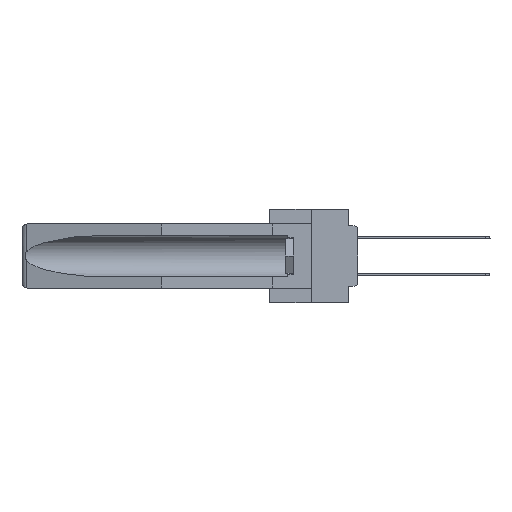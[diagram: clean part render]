
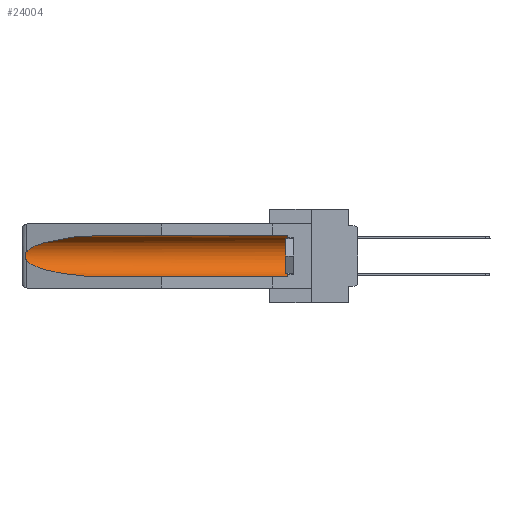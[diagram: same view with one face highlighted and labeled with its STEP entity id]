
A CAD part, left-side view. The second image highlights one B-rep face of the part: STEP entity #24004.
In plain terms, the highlighted cylindrical face has radius 2.857 mm (diameter 5.715 mm), a partial arc.
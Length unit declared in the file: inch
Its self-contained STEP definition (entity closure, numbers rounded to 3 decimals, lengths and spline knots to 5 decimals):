
#847 = CARTESIAN_POINT ( 'NONE',  ( 0.26537, 1.52718, -0.14972 ) ) ;
#1030 = CARTESIAN_POINT ( 'NONE',  ( 0.26654, 1.53092, -0.15636 ) ) ;
#1283 = CARTESIAN_POINT ( 'NONE',  ( 0.21114, 1.30732, -0.059 ) ) ;
#1475 = CARTESIAN_POINT ( 'NONE',  ( 0.2675, 1.53308, -0.16763 ) ) ;
#3165 = VERTEX_POINT ( 'NONE', #23333 ) ;
#3193 = DIRECTION ( 'NONE',  ( 0., 1., 0. ) ) ;
#3310 = B_SPLINE_CURVE_WITH_KNOTS ( 'NONE', 3,
 ( #15070, #26556, #1030, #21716, #1475, #8117, #28674, #17335, #8264, #5844 ),
 .UNSPECIFIED., .F., .F.,
 ( 4, 2, 2, 2, 4 ),
 ( 0., 0.00029, 0.00058, 0.00087, 0.00117 ),
 .UNSPECIFIED. ) ;
#3900 = CARTESIAN_POINT ( 'NONE',  ( 0.155, 0.126, -0.1715 ) ) ;
#3917 = CARTESIAN_POINT ( 'NONE',  ( 0.26537, 1.52718, -0.19328 ) ) ;
#4339 = VERTEX_POINT ( 'NONE', #29647 ) ;
#4673 = EDGE_CURVE ( 'NONE', #3165, #19928, #6039, .T. ) ;
#5576 = VECTOR ( 'NONE', #3193, 39.37008 ) ;
#5599 = VERTEX_POINT ( 'NONE', #15603 ) ;
#5844 = CARTESIAN_POINT ( 'NONE',  ( 0.26537, 1.52718, -0.19328 ) ) ;
#5873 = CARTESIAN_POINT ( 'NONE',  ( 0.25451, 1.48313, -0.24835 ) ) ;
#6039 = LINE ( 'NONE', #24465, #5576 ) ;
#6092 = FACE_OUTER_BOUND ( 'NONE', #16623, .T. ) ;
#7738 = ORIENTED_EDGE ( 'NONE', *, *, #23647, .T. ) ;
#7782 = CARTESIAN_POINT ( 'NONE',  ( 0.25451, 1.48313, -0.09465 ) ) ;
#7866 = VERTEX_POINT ( 'NONE', #18547 ) ;
#8006 = VERTEX_POINT ( 'NONE', #8987 ) ;
#8021 = ORIENTED_EDGE ( 'NONE', *, *, #13941, .F. ) ;
#8079 = DIRECTION ( 'NONE',  ( 0., 1., 0. ) ) ;
#8117 = CARTESIAN_POINT ( 'NONE',  ( 0.2675, 1.53308, -0.17534 ) ) ;
#8146 = CARTESIAN_POINT ( 'NONE',  ( 0.21114, 1.30732, -0.284 ) ) ;
#8264 = CARTESIAN_POINT ( 'NONE',  ( 0.26597, 1.5296, -0.19026 ) ) ;
#8423 = DIRECTION ( 'NONE',  ( 0., -1., 0. ) ) ;
#8987 = CARTESIAN_POINT ( 'NONE',  ( 0.155, 1.07973, -0.284 ) ) ;
#9455 = CARTESIAN_POINT ( 'NONE',  ( 0.155, -0.30754, -0.284 ) ) ;
#10213 = CARTESIAN_POINT ( 'NONE',  ( 0.155, 1.07973, -0.059 ) ) ;
#10490 = DIRECTION ( 'NONE',  ( 0., 0., 1. ) ) ;
#12015 = AXIS2_PLACEMENT_3D ( 'NONE', #3900, #8423, #17947 ) ;
#12179 = DIRECTION ( 'NONE',  ( 0., 1., 0. ) ) ;
#12548 = CARTESIAN_POINT ( 'NONE',  ( 0.155, 1.07973, -0.284 ) ) ;
#12677 = EDGE_CURVE ( 'NONE', #19928, #5599, #14949, .T. ) ;
#12957 = CIRCLE ( 'NONE', #12015, 0.1125 ) ;
#13941 = EDGE_CURVE ( 'NONE', #7866, #8006, #27748, .T. ) ;
#14568 = AXIS2_PLACEMENT_3D ( 'NONE', #29077, #8079, #10490 ) ;
#14949 =( BOUNDED_CURVE ( )  B_SPLINE_CURVE ( 3, ( #17151, #1283, #7782, #847 ),
 .UNSPECIFIED., .F., .F. ) 
 B_SPLINE_CURVE_WITH_KNOTS ( ( 4, 4 ),
 ( 4.71239, 6.08839 ),
 .UNSPECIFIED. ) 
 CURVE ( )  GEOMETRIC_REPRESENTATION_ITEM ( )  RATIONAL_B_SPLINE_CURVE ( ( 1., 0.848, 0.848, 1. ) ) 
 REPRESENTATION_ITEM ( '' )  );
#15070 = CARTESIAN_POINT ( 'NONE',  ( 0.26537, 1.52718, -0.14972 ) ) ;
#15603 = CARTESIAN_POINT ( 'NONE',  ( 0.26537, 1.52718, -0.14972 ) ) ;
#16623 = EDGE_LOOP ( 'NONE', ( #18403, #7738, #27579, #8021, #24237, #27445 ) ) ;
#17151 = CARTESIAN_POINT ( 'NONE',  ( 0.155, 1.07973, -0.059 ) ) ;
#17232 =( BOUNDED_CURVE ( )  B_SPLINE_CURVE ( 3, ( #3917, #5873, #8146, #12548 ),
 .UNSPECIFIED., .F., .F. ) 
 B_SPLINE_CURVE_WITH_KNOTS ( ( 4, 4 ),
 ( 0.1948, 1.5708 ),
 .UNSPECIFIED. ) 
 CURVE ( )  GEOMETRIC_REPRESENTATION_ITEM ( )  RATIONAL_B_SPLINE_CURVE ( ( 1., 0.848, 0.848, 1. ) ) 
 REPRESENTATION_ITEM ( '' )  );
#17335 = CARTESIAN_POINT ( 'NONE',  ( 0.26655, 1.53094, -0.18657 ) ) ;
#17947 = DIRECTION ( 'NONE',  ( 0., 0., 1. ) ) ;
#18403 = ORIENTED_EDGE ( 'NONE', *, *, #12677, .T. ) ;
#18547 = CARTESIAN_POINT ( 'NONE',  ( 0.155, 0.126, -0.284 ) ) ;
#19660 = EDGE_CURVE ( 'NONE', #7866, #3165, #12957, .T. ) ;
#19928 = VERTEX_POINT ( 'NONE', #10213 ) ;
#21716 = CARTESIAN_POINT ( 'NONE',  ( 0.2673, 1.5327, -0.16383 ) ) ;
#22085 = EDGE_CURVE ( 'NONE', #4339, #8006, #17232, .T. ) ;
#23333 = CARTESIAN_POINT ( 'NONE',  ( 0.155, 0.126, -0.059 ) ) ;
#23647 = EDGE_CURVE ( 'NONE', #5599, #4339, #3310, .T. ) ;
#24004 = ADVANCED_FACE ( 'NONE', ( #6092 ), #24085, .F. ) ;
#24085 = CYLINDRICAL_SURFACE ( 'NONE', #14568, 0.1125 ) ;
#24237 = ORIENTED_EDGE ( 'NONE', *, *, #19660, .T. ) ;
#24465 = CARTESIAN_POINT ( 'NONE',  ( 0.155, -0.30754, -0.059 ) ) ;
#26556 = CARTESIAN_POINT ( 'NONE',  ( 0.26597, 1.52961, -0.15275 ) ) ;
#26671 = VECTOR ( 'NONE', #12179, 39.37008 ) ;
#27445 = ORIENTED_EDGE ( 'NONE', *, *, #4673, .T. ) ;
#27579 = ORIENTED_EDGE ( 'NONE', *, *, #22085, .T. ) ;
#27748 = LINE ( 'NONE', #9455, #26671 ) ;
#28674 = CARTESIAN_POINT ( 'NONE',  ( 0.2673, 1.53269, -0.17917 ) ) ;
#29077 = CARTESIAN_POINT ( 'NONE',  ( 0.155, -0.30754, -0.1715 ) ) ;
#29647 = CARTESIAN_POINT ( 'NONE',  ( 0.26537, 1.52718, -0.19328 ) ) ;
